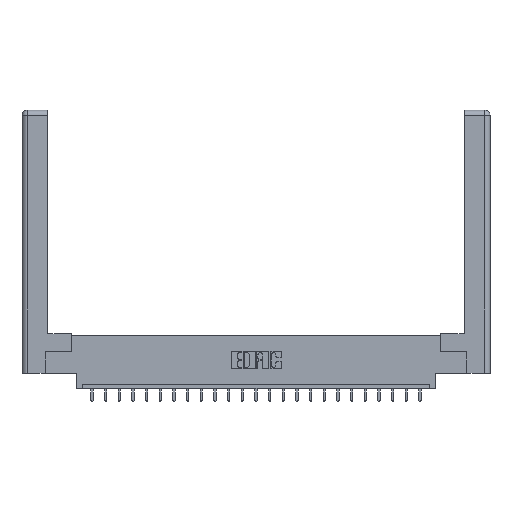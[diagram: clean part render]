
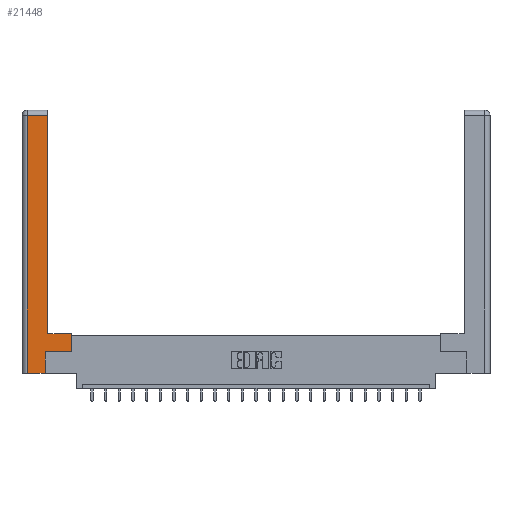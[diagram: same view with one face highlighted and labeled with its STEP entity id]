
A CAD part, top view. The second image highlights one B-rep face of the part: STEP entity #21448.
In plain terms, the highlighted planar face has unit normal (0, 0, 1).
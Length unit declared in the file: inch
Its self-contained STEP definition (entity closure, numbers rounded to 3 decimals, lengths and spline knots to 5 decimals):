
#633 = ORIENTED_EDGE ( 'NONE', *, *, #16893, .T. ) ;
#851 = LINE ( 'NONE', #1417, #21346 ) ;
#1245 = EDGE_CURVE ( 'NONE', #2738, #15262, #18783, .T. ) ;
#1417 = CARTESIAN_POINT ( 'NONE',  ( 0.565, 0.45, 0. ) ) ;
#2084 = CARTESIAN_POINT ( 'NONE',  ( 0.0615, 2.94, 0. ) ) ;
#2738 = VERTEX_POINT ( 'NONE', #2084 ) ;
#2900 = DIRECTION ( 'NONE',  ( 0., -1., 0. ) ) ;
#2969 = PLANE ( 'NONE',  #5106 ) ;
#3238 = VERTEX_POINT ( 'NONE', #21388 ) ;
#3316 = ORIENTED_EDGE ( 'NONE', *, *, #8247, .T. ) ;
#3385 = EDGE_CURVE ( 'NONE', #22908, #21779, #3862, .T. ) ;
#3419 = DIRECTION ( 'NONE',  ( -1., 0., 0. ) ) ;
#3603 = CARTESIAN_POINT ( 'NONE',  ( 0.265, 0.245, 0. ) ) ;
#3862 = LINE ( 'NONE', #3956, #6980 ) ;
#3956 = CARTESIAN_POINT ( 'NONE',  ( 0.265, 0.245, 0. ) ) ;
#4894 = DIRECTION ( 'NONE',  ( 1., 0., 0. ) ) ;
#5080 = CARTESIAN_POINT ( 'NONE',  ( 0.0615, 2.94, 0. ) ) ;
#5106 = AXIS2_PLACEMENT_3D ( 'NONE', #22767, #10111, #6469 ) ;
#5110 = VECTOR ( 'NONE', #2900, 39.37008 ) ;
#6100 = ORIENTED_EDGE ( 'NONE', *, *, #8888, .T. ) ;
#6469 = DIRECTION ( 'NONE',  ( -1., 0., 0. ) ) ;
#6645 = CARTESIAN_POINT ( 'NONE',  ( 0.265, 0., 0. ) ) ;
#6781 = EDGE_CURVE ( 'NONE', #21636, #19539, #851, .T. ) ;
#6822 = LINE ( 'NONE', #5080, #15950 ) ;
#6917 = EDGE_CURVE ( 'NONE', #15262, #22908, #19639, .T. ) ;
#6926 = ORIENTED_EDGE ( 'NONE', *, *, #1245, .T. ) ;
#6980 = VECTOR ( 'NONE', #20574, 39.37008 ) ;
#7449 = CARTESIAN_POINT ( 'NONE',  ( 0.265, 0., 0. ) ) ;
#7705 = DIRECTION ( 'NONE',  ( -1., 0., 0. ) ) ;
#8035 = CARTESIAN_POINT ( 'NONE',  ( 0.295, 0.45, 0. ) ) ;
#8247 = EDGE_CURVE ( 'NONE', #19539, #13004, #14744, .T. ) ;
#8888 = EDGE_CURVE ( 'NONE', #21779, #21636, #20120, .T. ) ;
#8960 = CARTESIAN_POINT ( 'NONE',  ( 0.295, 3., 0. ) ) ;
#9507 = ORIENTED_EDGE ( 'NONE', *, *, #3385, .T. ) ;
#9606 = VECTOR ( 'NONE', #7705, 39.37008 ) ;
#10111 = DIRECTION ( 'NONE',  ( 0., 0., -1. ) ) ;
#10133 = CARTESIAN_POINT ( 'NONE',  ( 0.0615, 0., 0. ) ) ;
#10322 = ORIENTED_EDGE ( 'NONE', *, *, #6781, .T. ) ;
#10760 = DIRECTION ( 'NONE',  ( 0., 1., 0. ) ) ;
#12019 = ORIENTED_EDGE ( 'NONE', *, *, #22317, .T. ) ;
#13004 = VERTEX_POINT ( 'NONE', #20601 ) ;
#13591 = VECTOR ( 'NONE', #10760, 39.37008 ) ;
#13750 = ORIENTED_EDGE ( 'NONE', *, *, #6917, .T. ) ;
#14744 = LINE ( 'NONE', #8035, #9606 ) ;
#15262 = VERTEX_POINT ( 'NONE', #20404 ) ;
#15950 = VECTOR ( 'NONE', #3419, 39.37008 ) ;
#16538 = DIRECTION ( 'NONE',  ( 1., 0., 0. ) ) ;
#16893 = EDGE_CURVE ( 'NONE', #13004, #3238, #17872, .T. ) ;
#17130 = FACE_OUTER_BOUND ( 'NONE', #23100, .T. ) ;
#17674 = CARTESIAN_POINT ( 'NONE',  ( 0.565, 0.45, 0. ) ) ;
#17872 = LINE ( 'NONE', #8960, #13591 ) ;
#18783 = LINE ( 'NONE', #10133, #5110 ) ;
#19539 = VERTEX_POINT ( 'NONE', #17674 ) ;
#19639 = LINE ( 'NONE', #7449, #22196 ) ;
#19692 = CARTESIAN_POINT ( 'NONE',  ( 0.565, 0.245, 0. ) ) ;
#19796 = DIRECTION ( 'NONE',  ( 0., 1., 0. ) ) ;
#20120 = LINE ( 'NONE', #19692, #22970 ) ;
#20404 = CARTESIAN_POINT ( 'NONE',  ( 0.0615, 0., 0. ) ) ;
#20574 = DIRECTION ( 'NONE',  ( 0., 1., 0. ) ) ;
#20601 = CARTESIAN_POINT ( 'NONE',  ( 0.295, 0.45, 0. ) ) ;
#21346 = VECTOR ( 'NONE', #19796, 39.37008 ) ;
#21388 = CARTESIAN_POINT ( 'NONE',  ( 0.295, 2.94, 0. ) ) ;
#21448 = ADVANCED_FACE ( 'NONE', ( #17130 ), #2969, .F. ) ;
#21636 = VERTEX_POINT ( 'NONE', #21651 ) ;
#21651 = CARTESIAN_POINT ( 'NONE',  ( 0.565, 0.245, 0. ) ) ;
#21779 = VERTEX_POINT ( 'NONE', #3603 ) ;
#22196 = VECTOR ( 'NONE', #16538, 39.37008 ) ;
#22317 = EDGE_CURVE ( 'NONE', #3238, #2738, #6822, .T. ) ;
#22767 = CARTESIAN_POINT ( 'NONE',  ( 0., 0., 0. ) ) ;
#22908 = VERTEX_POINT ( 'NONE', #6645 ) ;
#22970 = VECTOR ( 'NONE', #4894, 39.37008 ) ;
#23100 = EDGE_LOOP ( 'NONE', ( #633, #12019, #6926, #13750, #9507, #6100, #10322, #3316 ) ) ;
